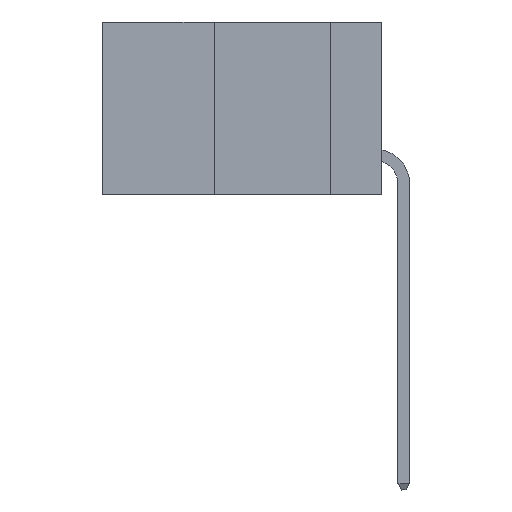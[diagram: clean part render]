
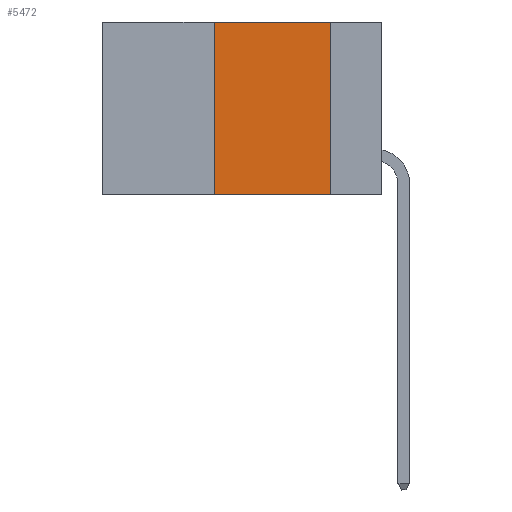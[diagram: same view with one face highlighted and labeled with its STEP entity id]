
A CAD part, left-side view. The second image highlights one B-rep face of the part: STEP entity #5472.
In plain terms, the highlighted planar face has unit normal (-1, 0, 0).
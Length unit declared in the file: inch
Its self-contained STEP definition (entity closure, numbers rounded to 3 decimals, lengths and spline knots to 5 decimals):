
#1142 = LINE ( 'NONE', #7838, #19929 ) ;
#1575 = EDGE_CURVE ( 'NONE', #21110, #9434, #1142, .T. ) ;
#2727 = EDGE_LOOP ( 'NONE', ( #2784, #20689, #3298, #4042 ) ) ;
#2784 = ORIENTED_EDGE ( 'NONE', *, *, #1575, .F. ) ;
#3298 = ORIENTED_EDGE ( 'NONE', *, *, #17187, .F. ) ;
#3401 = DIRECTION ( 'NONE',  ( 0., 0., 1. ) ) ;
#3615 = EDGE_CURVE ( 'NONE', #19911, #21110, #19550, .T. ) ;
#4042 = ORIENTED_EDGE ( 'NONE', *, *, #20941, .T. ) ;
#5472 = ADVANCED_FACE ( 'NONE', ( #12942 ), #7218, .F. ) ;
#5597 = CARTESIAN_POINT ( 'NONE',  ( 0., 0.6, 0. ) ) ;
#6388 = DIRECTION ( 'NONE',  ( 0., 0., -1. ) ) ;
#7218 = PLANE ( 'NONE',  #10254 ) ;
#7838 = CARTESIAN_POINT ( 'NONE',  ( 0., 0.11, 0. ) ) ;
#8841 = CARTESIAN_POINT ( 'NONE',  ( 0., 0.36, -0.37 ) ) ;
#9434 = VERTEX_POINT ( 'NONE', #11397 ) ;
#10254 = AXIS2_PLACEMENT_3D ( 'NONE', #5597, #17594, #14214 ) ;
#10806 = VECTOR ( 'NONE', #14018, 39.37008 ) ;
#10874 = CARTESIAN_POINT ( 'NONE',  ( 0., 0.11, 0. ) ) ;
#11397 = CARTESIAN_POINT ( 'NONE',  ( 0., 0.11, -0.37 ) ) ;
#12942 = FACE_OUTER_BOUND ( 'NONE', #2727, .T. ) ;
#13579 = VECTOR ( 'NONE', #17352, 39.37008 ) ;
#14018 = DIRECTION ( 'NONE',  ( 0., -1., 0. ) ) ;
#14053 = VECTOR ( 'NONE', #3401, 39.37008 ) ;
#14214 = DIRECTION ( 'NONE',  ( 0., 0., -1. ) ) ;
#15414 = LINE ( 'NONE', #16951, #10806 ) ;
#16448 = LINE ( 'NONE', #17132, #14053 ) ;
#16951 = CARTESIAN_POINT ( 'NONE',  ( 0., 0.6, -0.37 ) ) ;
#17132 = CARTESIAN_POINT ( 'NONE',  ( 0., 0.36, 0. ) ) ;
#17187 = EDGE_CURVE ( 'NONE', #20439, #19911, #16448, .T. ) ;
#17352 = DIRECTION ( 'NONE',  ( 0., -1., 0. ) ) ;
#17586 = CARTESIAN_POINT ( 'NONE',  ( 0., 0.36, 0. ) ) ;
#17594 = DIRECTION ( 'NONE',  ( 1., 0., 0. ) ) ;
#19550 = LINE ( 'NONE', #22477, #13579 ) ;
#19911 = VERTEX_POINT ( 'NONE', #17586 ) ;
#19929 = VECTOR ( 'NONE', #6388, 39.37008 ) ;
#20439 = VERTEX_POINT ( 'NONE', #8841 ) ;
#20689 = ORIENTED_EDGE ( 'NONE', *, *, #3615, .F. ) ;
#20941 = EDGE_CURVE ( 'NONE', #20439, #9434, #15414, .T. ) ;
#21110 = VERTEX_POINT ( 'NONE', #10874 ) ;
#22477 = CARTESIAN_POINT ( 'NONE',  ( 0., 0.6, 0. ) ) ;
